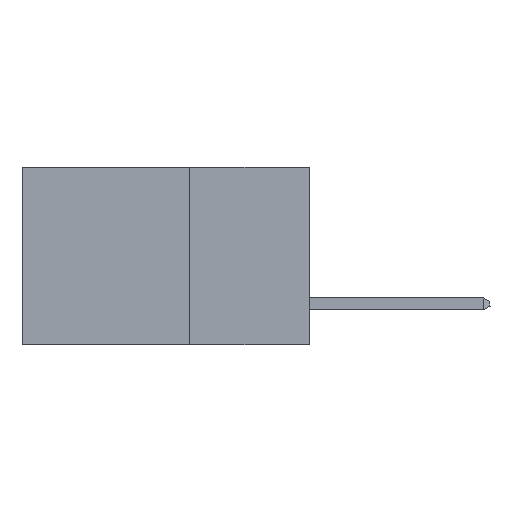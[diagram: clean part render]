
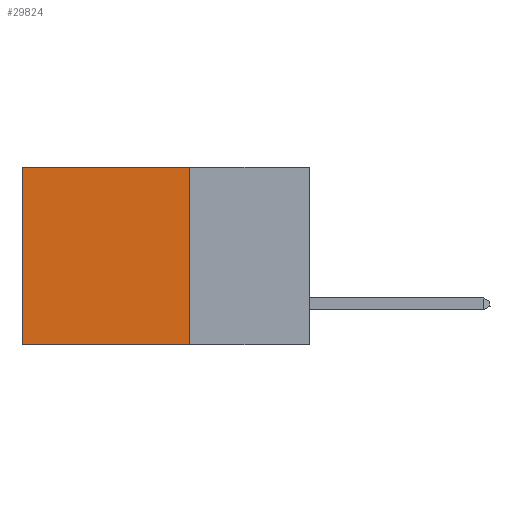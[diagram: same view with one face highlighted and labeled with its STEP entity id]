
A CAD part, left-side view. The second image highlights one B-rep face of the part: STEP entity #29824.
In plain terms, the highlighted planar face has unit normal (-1, 0, 0).
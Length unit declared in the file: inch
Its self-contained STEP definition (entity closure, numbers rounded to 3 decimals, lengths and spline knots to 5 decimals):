
#3085 = EDGE_CURVE ( 'NONE', #22497, #33370, #21699, .T. ) ;
#3331 = EDGE_CURVE ( 'NONE', #33370, #8446, #9620, .T. ) ;
#4186 = DIRECTION ( 'NONE',  ( 0., 1., 0. ) ) ;
#4464 = ORIENTED_EDGE ( 'NONE', *, *, #6468, .F. ) ;
#6201 = LINE ( 'NONE', #42463, #14353 ) ;
#6468 = EDGE_CURVE ( 'NONE', #22497, #11021, #19761, .T. ) ;
#8446 = VERTEX_POINT ( 'NONE', #21993 ) ;
#9620 = LINE ( 'NONE', #44714, #24399 ) ;
#10765 = PLANE ( 'NONE',  #39316 ) ;
#10985 = VECTOR ( 'NONE', #30913, 39.37008 ) ;
#11021 = VERTEX_POINT ( 'NONE', #27298 ) ;
#14353 = VECTOR ( 'NONE', #4186, 39.37008 ) ;
#14556 = DIRECTION ( 'NONE',  ( 1., 0., 0. ) ) ;
#15204 = EDGE_LOOP ( 'NONE', ( #19983, #15761, #4464, #31393 ) ) ;
#15761 = ORIENTED_EDGE ( 'NONE', *, *, #36416, .F. ) ;
#16325 = CARTESIAN_POINT ( 'NONE',  ( 0.2875, 0.25, 0. ) ) ;
#19761 = LINE ( 'NONE', #34418, #10985 ) ;
#19983 = ORIENTED_EDGE ( 'NONE', *, *, #3331, .T. ) ;
#21699 = LINE ( 'NONE', #31425, #36384 ) ;
#21993 = CARTESIAN_POINT ( 'NONE',  ( 0.2875, 0.6, -0.37 ) ) ;
#22497 = VERTEX_POINT ( 'NONE', #16325 ) ;
#24399 = VECTOR ( 'NONE', #41065, 39.37008 ) ;
#27298 = CARTESIAN_POINT ( 'NONE',  ( 0.2875, 0.25, -0.37 ) ) ;
#29824 = ADVANCED_FACE ( 'NONE', ( #37082 ), #10765, .F. ) ;
#30397 = CARTESIAN_POINT ( 'NONE',  ( 0.2875, 0.6, 0. ) ) ;
#30913 = DIRECTION ( 'NONE',  ( 0., 0., -1. ) ) ;
#31393 = ORIENTED_EDGE ( 'NONE', *, *, #3085, .T. ) ;
#31425 = CARTESIAN_POINT ( 'NONE',  ( 0.2875, 0.25, 0. ) ) ;
#33370 = VERTEX_POINT ( 'NONE', #30397 ) ;
#34418 = CARTESIAN_POINT ( 'NONE',  ( 0.2875, 0.25, 0. ) ) ;
#35512 = CARTESIAN_POINT ( 'NONE',  ( 0.2875, 0.25, 0. ) ) ;
#36384 = VECTOR ( 'NONE', #39328, 39.37008 ) ;
#36416 = EDGE_CURVE ( 'NONE', #11021, #8446, #6201, .T. ) ;
#37082 = FACE_OUTER_BOUND ( 'NONE', #15204, .T. ) ;
#38371 = DIRECTION ( 'NONE',  ( 0., 0., -1. ) ) ;
#39316 = AXIS2_PLACEMENT_3D ( 'NONE', #35512, #14556, #38371 ) ;
#39328 = DIRECTION ( 'NONE',  ( 0., 1., 0. ) ) ;
#41065 = DIRECTION ( 'NONE',  ( 0., 0., -1. ) ) ;
#42463 = CARTESIAN_POINT ( 'NONE',  ( 0.2875, 0.25, -0.37 ) ) ;
#44714 = CARTESIAN_POINT ( 'NONE',  ( 0.2875, 0.6, 0. ) ) ;
